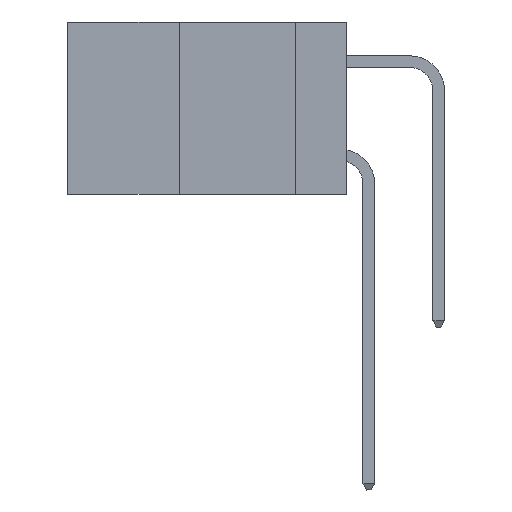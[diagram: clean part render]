
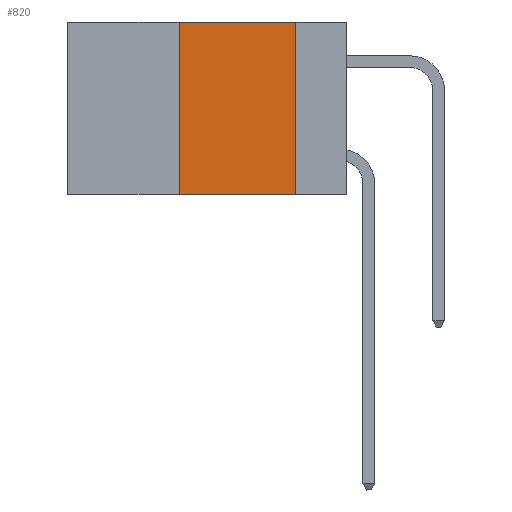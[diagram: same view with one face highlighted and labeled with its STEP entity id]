
A CAD part, left-side view. The second image highlights one B-rep face of the part: STEP entity #820.
In plain terms, the highlighted planar face has unit normal (-1, 0, 0).
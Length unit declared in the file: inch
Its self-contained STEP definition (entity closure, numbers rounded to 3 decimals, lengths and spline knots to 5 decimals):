
#127 = ORIENTED_EDGE ( 'NONE', *, *, #10605, .F. ) ;
#290 = ORIENTED_EDGE ( 'NONE', *, *, #3280, .T. ) ;
#764 = DIRECTION ( 'NONE',  ( 0., 0., 1. ) ) ;
#820 = ADVANCED_FACE ( 'NONE', ( #10754 ), #5742, .F. ) ;
#850 = CARTESIAN_POINT ( 'NONE',  ( 0., 0.11, 0. ) ) ;
#1551 = VERTEX_POINT ( 'NONE', #12374 ) ;
#2869 = CARTESIAN_POINT ( 'NONE',  ( 0., 0.11, -0.37 ) ) ;
#3116 = DIRECTION ( 'NONE',  ( 0., -1., 0. ) ) ;
#3230 = DIRECTION ( 'NONE',  ( 0., 0., -1. ) ) ;
#3280 = EDGE_CURVE ( 'NONE', #1551, #13858, #5544, .T. ) ;
#3541 = VECTOR ( 'NONE', #764, 39.37008 ) ;
#3635 = DIRECTION ( 'NONE',  ( 0., 0., -1. ) ) ;
#4156 = ORIENTED_EDGE ( 'NONE', *, *, #12217, .F. ) ;
#4800 = ORIENTED_EDGE ( 'NONE', *, *, #12328, .F. ) ;
#5059 = DIRECTION ( 'NONE',  ( 1., 0., 0. ) ) ;
#5351 = AXIS2_PLACEMENT_3D ( 'NONE', #7283, #5059, #3635 ) ;
#5480 = VECTOR ( 'NONE', #13922, 39.37008 ) ;
#5544 = LINE ( 'NONE', #13465, #11227 ) ;
#5678 = VERTEX_POINT ( 'NONE', #850 ) ;
#5742 = PLANE ( 'NONE',  #5351 ) ;
#7283 = CARTESIAN_POINT ( 'NONE',  ( 0., 0.6, 0. ) ) ;
#7470 = EDGE_LOOP ( 'NONE', ( #127, #4800, #4156, #290 ) ) ;
#7715 = CARTESIAN_POINT ( 'NONE',  ( 0., 0.11, 0. ) ) ;
#8376 = LINE ( 'NONE', #8846, #5480 ) ;
#8529 = CARTESIAN_POINT ( 'NONE',  ( 0., 0.36, 0. ) ) ;
#8846 = CARTESIAN_POINT ( 'NONE',  ( 0., 0.6, 0. ) ) ;
#8906 = CARTESIAN_POINT ( 'NONE',  ( 0., 0.36, 0. ) ) ;
#10605 = EDGE_CURVE ( 'NONE', #5678, #13858, #11361, .T. ) ;
#10754 = FACE_OUTER_BOUND ( 'NONE', #7470, .T. ) ;
#11227 = VECTOR ( 'NONE', #3116, 39.37008 ) ;
#11361 = LINE ( 'NONE', #7715, #11996 ) ;
#11814 = VERTEX_POINT ( 'NONE', #8906 ) ;
#11996 = VECTOR ( 'NONE', #3230, 39.37008 ) ;
#12131 = LINE ( 'NONE', #8529, #3541 ) ;
#12217 = EDGE_CURVE ( 'NONE', #1551, #11814, #12131, .T. ) ;
#12328 = EDGE_CURVE ( 'NONE', #11814, #5678, #8376, .T. ) ;
#12374 = CARTESIAN_POINT ( 'NONE',  ( 0., 0.36, -0.37 ) ) ;
#13465 = CARTESIAN_POINT ( 'NONE',  ( 0., 0.6, -0.37 ) ) ;
#13858 = VERTEX_POINT ( 'NONE', #2869 ) ;
#13922 = DIRECTION ( 'NONE',  ( 0., -1., 0. ) ) ;
